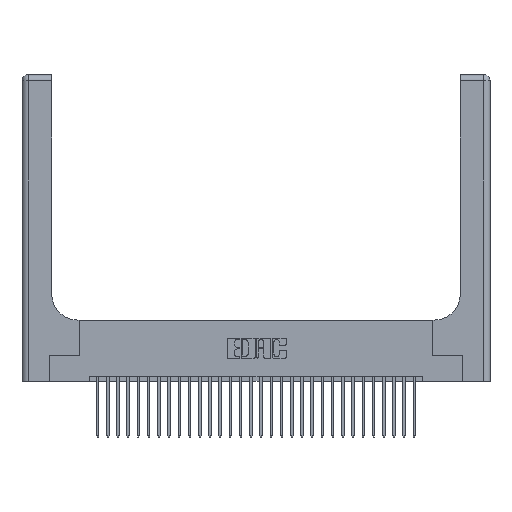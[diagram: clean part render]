
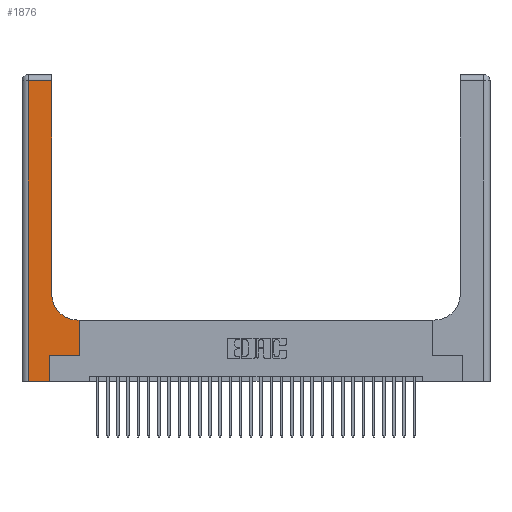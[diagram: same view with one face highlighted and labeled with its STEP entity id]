
A CAD part, top view. The second image highlights one B-rep face of the part: STEP entity #1876.
In plain terms, the highlighted planar face has unit normal (0, 0, 1).
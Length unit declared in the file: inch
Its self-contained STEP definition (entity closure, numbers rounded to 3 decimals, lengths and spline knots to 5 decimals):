
#209 = CARTESIAN_POINT ( 'NONE',  ( 0.269, 0., 0.37 ) ) ;
#225 = ORIENTED_EDGE ( 'NONE', *, *, #1005, .T. ) ;
#643 = VECTOR ( 'NONE', #6510, 39.37008 ) ;
#778 = CARTESIAN_POINT ( 'NONE',  ( 0.06, 0., 0.37 ) ) ;
#1005 = EDGE_CURVE ( 'NONE', #30688, #6284, #19071, .T. ) ;
#1406 = VECTOR ( 'NONE', #12511, 39.37008 ) ;
#1471 = CARTESIAN_POINT ( 'NONE',  ( 0.5585, 0.25, 0.37 ) ) ;
#1876 = ADVANCED_FACE ( 'NONE', ( #27811 ), #4809, .F. ) ;
#1940 = VECTOR ( 'NONE', #25112, 39.37008 ) ;
#2015 = CARTESIAN_POINT ( 'NONE',  ( 0.269, 0.25, 0.37 ) ) ;
#2244 = EDGE_LOOP ( 'NONE', ( #28151, #28058, #22197, #14631, #21751, #20754, #22884, #23416, #225 ) ) ;
#2379 = VECTOR ( 'NONE', #8495, 39.37008 ) ;
#2656 = EDGE_CURVE ( 'NONE', #10422, #30526, #14068, .T. ) ;
#2876 = EDGE_CURVE ( 'NONE', #22459, #17515, #7962, .T. ) ;
#4809 = PLANE ( 'NONE',  #6393 ) ;
#6219 = VECTOR ( 'NONE', #31433, 39.37008 ) ;
#6284 = VERTEX_POINT ( 'NONE', #20537 ) ;
#6393 = AXIS2_PLACEMENT_3D ( 'NONE', #21942, #24372, #9748 ) ;
#6510 = DIRECTION ( 'NONE',  ( 0., -1., 0. ) ) ;
#7169 = LINE ( 'NONE', #21161, #643 ) ;
#7300 = VECTOR ( 'NONE', #28908, 39.37008 ) ;
#7554 = EDGE_CURVE ( 'NONE', #30526, #22459, #15416, .T. ) ;
#7876 = EDGE_CURVE ( 'NONE', #6284, #29419, #12727, .T. ) ;
#7915 = DIRECTION ( 'NONE',  ( 0., 1., 0. ) ) ;
#7962 = LINE ( 'NONE', #27118, #1406 ) ;
#8076 = LINE ( 'NONE', #9369, #7300 ) ;
#8495 = DIRECTION ( 'NONE',  ( 1., 0., 0. ) ) ;
#8542 = VECTOR ( 'NONE', #15632, 39.37008 ) ;
#8847 = DIRECTION ( 'NONE',  ( 0., 0., -1. ) ) ;
#9369 = CARTESIAN_POINT ( 'NONE',  ( 0.2915, 0.6, 0.37 ) ) ;
#9748 = DIRECTION ( 'NONE',  ( -1., 0., 0. ) ) ;
#10422 = VERTEX_POINT ( 'NONE', #209 ) ;
#11349 = EDGE_CURVE ( 'NONE', #17515, #30688, #8076, .T. ) ;
#11700 = VERTEX_POINT ( 'NONE', #778 ) ;
#12511 = DIRECTION ( 'NONE',  ( 0., 1., 0. ) ) ;
#12646 = CARTESIAN_POINT ( 'NONE',  ( 0.06, 2.94, 0.37 ) ) ;
#12727 = LINE ( 'NONE', #26498, #6219 ) ;
#13128 = AXIS2_PLACEMENT_3D ( 'NONE', #23475, #8847, #25917 ) ;
#14068 = LINE ( 'NONE', #29794, #26277 ) ;
#14631 = ORIENTED_EDGE ( 'NONE', *, *, #25610, .T. ) ;
#15416 = LINE ( 'NONE', #15739, #2379 ) ;
#15632 = DIRECTION ( 'NONE',  ( -1., 0., 0. ) ) ;
#15739 = CARTESIAN_POINT ( 'NONE',  ( 0.269, 0.25, 0.37 ) ) ;
#16362 = VERTEX_POINT ( 'NONE', #12646 ) ;
#17515 = VERTEX_POINT ( 'NONE', #19639 ) ;
#19071 = CIRCLE ( 'NONE', #13128, 0.25 ) ;
#19462 = EDGE_CURVE ( 'NONE', #29419, #16362, #20772, .T. ) ;
#19639 = CARTESIAN_POINT ( 'NONE',  ( 0.5585, 0.6, 0.37 ) ) ;
#19802 = CARTESIAN_POINT ( 'NONE',  ( 0.5415, 0.6, 0.37 ) ) ;
#20537 = CARTESIAN_POINT ( 'NONE',  ( 0.2915, 0.85, 0.37 ) ) ;
#20569 = CARTESIAN_POINT ( 'NONE',  ( 0., 2.94, 0.37 ) ) ;
#20717 = LINE ( 'NONE', #22674, #1940 ) ;
#20754 = ORIENTED_EDGE ( 'NONE', *, *, #7554, .T. ) ;
#20772 = LINE ( 'NONE', #20569, #8542 ) ;
#21161 = CARTESIAN_POINT ( 'NONE',  ( 0.06, 3., 0.37 ) ) ;
#21751 = ORIENTED_EDGE ( 'NONE', *, *, #2656, .T. ) ;
#21942 = CARTESIAN_POINT ( 'NONE',  ( 0., 3., 0.37 ) ) ;
#22197 = ORIENTED_EDGE ( 'NONE', *, *, #28825, .T. ) ;
#22459 = VERTEX_POINT ( 'NONE', #1471 ) ;
#22674 = CARTESIAN_POINT ( 'NONE',  ( 0., 0., 0.37 ) ) ;
#22884 = ORIENTED_EDGE ( 'NONE', *, *, #2876, .T. ) ;
#23416 = ORIENTED_EDGE ( 'NONE', *, *, #11349, .T. ) ;
#23475 = CARTESIAN_POINT ( 'NONE',  ( 0.5415, 0.85, 0.37 ) ) ;
#24372 = DIRECTION ( 'NONE',  ( 0., 0., -1. ) ) ;
#25112 = DIRECTION ( 'NONE',  ( 1., 0., 0. ) ) ;
#25610 = EDGE_CURVE ( 'NONE', #11700, #10422, #20717, .T. ) ;
#25917 = DIRECTION ( 'NONE',  ( 1., 0., 0. ) ) ;
#26277 = VECTOR ( 'NONE', #7915, 39.37008 ) ;
#26498 = CARTESIAN_POINT ( 'NONE',  ( 0.2915, 3., 0.37 ) ) ;
#26876 = CARTESIAN_POINT ( 'NONE',  ( 0.2915, 2.94, 0.37 ) ) ;
#27118 = CARTESIAN_POINT ( 'NONE',  ( 0.5585, 0.25, 0.37 ) ) ;
#27811 = FACE_OUTER_BOUND ( 'NONE', #2244, .T. ) ;
#28058 = ORIENTED_EDGE ( 'NONE', *, *, #19462, .T. ) ;
#28151 = ORIENTED_EDGE ( 'NONE', *, *, #7876, .T. ) ;
#28825 = EDGE_CURVE ( 'NONE', #16362, #11700, #7169, .T. ) ;
#28908 = DIRECTION ( 'NONE',  ( -1., 0., 0. ) ) ;
#29419 = VERTEX_POINT ( 'NONE', #26876 ) ;
#29794 = CARTESIAN_POINT ( 'NONE',  ( 0.269, 0., 0.37 ) ) ;
#30526 = VERTEX_POINT ( 'NONE', #2015 ) ;
#30688 = VERTEX_POINT ( 'NONE', #19802 ) ;
#31433 = DIRECTION ( 'NONE',  ( 0., 1., 0. ) ) ;
